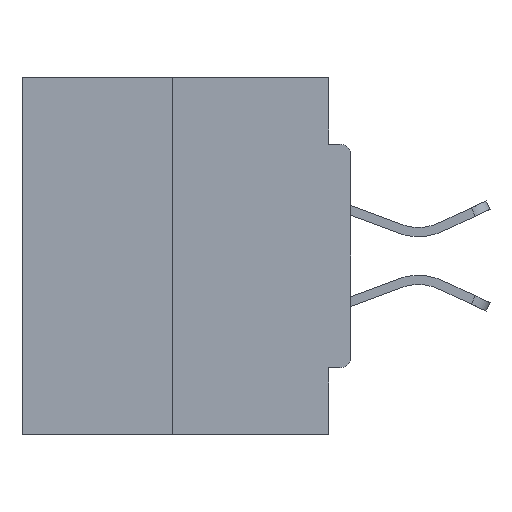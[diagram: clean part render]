
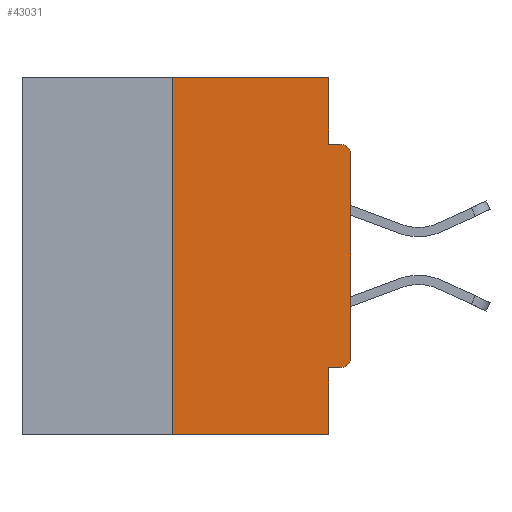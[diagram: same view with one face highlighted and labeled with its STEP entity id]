
A CAD part, left-side view. The second image highlights one B-rep face of the part: STEP entity #43031.
In plain terms, the highlighted planar face has unit normal (-1, 0, 0).
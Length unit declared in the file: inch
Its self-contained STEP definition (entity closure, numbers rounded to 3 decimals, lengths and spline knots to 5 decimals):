
#388 = EDGE_CURVE ( 'NONE', #30158, #618, #37627, .T. ) ;
#589 = EDGE_LOOP ( 'NONE', ( #16905, #14267, #35925, #22014, #29680, #1202, #29172, #22829, #21904, #15482 ) ) ;
#618 = VERTEX_POINT ( 'NONE', #36093 ) ;
#1078 = DIRECTION ( 'NONE',  ( 0., 0., -1. ) ) ;
#1202 = ORIENTED_EDGE ( 'NONE', *, *, #42570, .T. ) ;
#1735 = DIRECTION ( 'NONE',  ( 0., 1., 0. ) ) ;
#2717 = VERTEX_POINT ( 'NONE', #10126 ) ;
#3040 = VECTOR ( 'NONE', #42446, 39.37008 ) ;
#4078 = LINE ( 'NONE', #16279, #25141 ) ;
#4803 = DIRECTION ( 'NONE',  ( 0., 0., 1. ) ) ;
#5194 = CARTESIAN_POINT ( 'NONE',  ( 0., 0.031, -0.5 ) ) ;
#5253 = VERTEX_POINT ( 'NONE', #21710 ) ;
#5797 = VECTOR ( 'NONE', #20323, 39.37008 ) ;
#6685 = AXIS2_PLACEMENT_3D ( 'NONE', #8991, #26869, #28154 ) ;
#8008 = DIRECTION ( 'NONE',  ( -1., 0., 0. ) ) ;
#8043 = EDGE_CURVE ( 'NONE', #33575, #43270, #4078, .T. ) ;
#8541 = AXIS2_PLACEMENT_3D ( 'NONE', #38069, #44558, #27906 ) ;
#8991 = CARTESIAN_POINT ( 'NONE',  ( 0., 0.46, 0. ) ) ;
#9276 = CARTESIAN_POINT ( 'NONE',  ( 0., 0.031, 0. ) ) ;
#9399 = FACE_OUTER_BOUND ( 'NONE', #589, .T. ) ;
#9780 = DIRECTION ( 'NONE',  ( 0., -1., 0. ) ) ;
#10126 = CARTESIAN_POINT ( 'NONE',  ( 0., 0.031, 0. ) ) ;
#10431 = VECTOR ( 'NONE', #30221, 39.37008 ) ;
#10595 = VECTOR ( 'NONE', #38241, 39.37008 ) ;
#11610 = CARTESIAN_POINT ( 'NONE',  ( 0., 0., 0. ) ) ;
#12205 = CARTESIAN_POINT ( 'NONE',  ( 0., 0.25, -0.5 ) ) ;
#12233 = EDGE_CURVE ( 'NONE', #35413, #2717, #32429, .T. ) ;
#13070 = CARTESIAN_POINT ( 'NONE',  ( 0., 0.25, 0. ) ) ;
#14076 = CARTESIAN_POINT ( 'NONE',  ( 0., 0.031, -0.5 ) ) ;
#14267 = ORIENTED_EDGE ( 'NONE', *, *, #23577, .F. ) ;
#15436 = LINE ( 'NONE', #14076, #10595 ) ;
#15482 = ORIENTED_EDGE ( 'NONE', *, *, #19697, .F. ) ;
#15770 = CARTESIAN_POINT ( 'NONE',  ( 0., 0., -0.3915 ) ) ;
#16279 = CARTESIAN_POINT ( 'NONE',  ( 0., 0.46, -0.5 ) ) ;
#16905 = ORIENTED_EDGE ( 'NONE', *, *, #12233, .F. ) ;
#17288 = CIRCLE ( 'NONE', #37635, 0.015 ) ;
#17863 = VERTEX_POINT ( 'NONE', #33842 ) ;
#18727 = CARTESIAN_POINT ( 'NONE',  ( 0., 0.015, -0.3915 ) ) ;
#18904 = CARTESIAN_POINT ( 'NONE',  ( 0., 0.031, -0.0935 ) ) ;
#19132 = CARTESIAN_POINT ( 'NONE',  ( 0., 0.46, 0. ) ) ;
#19697 = EDGE_CURVE ( 'NONE', #2717, #30158, #44481, .T. ) ;
#20171 = CARTESIAN_POINT ( 'NONE',  ( 0., 0.015, -0.4065 ) ) ;
#20323 = DIRECTION ( 'NONE',  ( 0., 0., 1. ) ) ;
#21710 = CARTESIAN_POINT ( 'NONE',  ( 0., 0.031, -0.4065 ) ) ;
#21904 = ORIENTED_EDGE ( 'NONE', *, *, #388, .F. ) ;
#22014 = ORIENTED_EDGE ( 'NONE', *, *, #27966, .F. ) ;
#22829 = ORIENTED_EDGE ( 'NONE', *, *, #36757, .T. ) ;
#23577 = EDGE_CURVE ( 'NONE', #33575, #35413, #40900, .T. ) ;
#24592 = VERTEX_POINT ( 'NONE', #15770 ) ;
#25141 = VECTOR ( 'NONE', #9780, 39.37008 ) ;
#26398 = EDGE_CURVE ( 'NONE', #24592, #17863, #41490, .T. ) ;
#26869 = DIRECTION ( 'NONE',  ( 1., 0., 0. ) ) ;
#27906 = DIRECTION ( 'NONE',  ( 0., 0., -1. ) ) ;
#27966 = EDGE_CURVE ( 'NONE', #5253, #43270, #15436, .T. ) ;
#28154 = DIRECTION ( 'NONE',  ( 0., 0., -1. ) ) ;
#29172 = ORIENTED_EDGE ( 'NONE', *, *, #26398, .T. ) ;
#29680 = ORIENTED_EDGE ( 'NONE', *, *, #35485, .F. ) ;
#30158 = VERTEX_POINT ( 'NONE', #18904 ) ;
#30221 = DIRECTION ( 'NONE',  ( 0., 0., -1. ) ) ;
#31875 = CARTESIAN_POINT ( 'NONE',  ( 0., 0.25, 0. ) ) ;
#32097 = VECTOR ( 'NONE', #1735, 39.37008 ) ;
#32429 = LINE ( 'NONE', #19132, #40568 ) ;
#33575 = VERTEX_POINT ( 'NONE', #12205 ) ;
#33842 = CARTESIAN_POINT ( 'NONE',  ( 0., 0., -0.1085 ) ) ;
#35409 = LINE ( 'NONE', #39925, #32097 ) ;
#35413 = VERTEX_POINT ( 'NONE', #31875 ) ;
#35485 = EDGE_CURVE ( 'NONE', #40010, #5253, #35409, .T. ) ;
#35925 = ORIENTED_EDGE ( 'NONE', *, *, #8043, .T. ) ;
#36093 = CARTESIAN_POINT ( 'NONE',  ( 0., 0.015, -0.0935 ) ) ;
#36757 = EDGE_CURVE ( 'NONE', #17863, #618, #37456, .T. ) ;
#37456 = CIRCLE ( 'NONE', #8541, 0.015 ) ;
#37627 = LINE ( 'NONE', #42755, #3040 ) ;
#37635 = AXIS2_PLACEMENT_3D ( 'NONE', #18727, #8008, #1078 ) ;
#38069 = CARTESIAN_POINT ( 'NONE',  ( 0., 0.015, -0.1085 ) ) ;
#38241 = DIRECTION ( 'NONE',  ( 0., 0., -1. ) ) ;
#39925 = CARTESIAN_POINT ( 'NONE',  ( 0., 0., -0.4065 ) ) ;
#40010 = VERTEX_POINT ( 'NONE', #20171 ) ;
#40413 = VECTOR ( 'NONE', #4803, 39.37008 ) ;
#40568 = VECTOR ( 'NONE', #43400, 39.37008 ) ;
#40900 = LINE ( 'NONE', #13070, #5797 ) ;
#41490 = LINE ( 'NONE', #11610, #40413 ) ;
#42434 = PLANE ( 'NONE',  #6685 ) ;
#42446 = DIRECTION ( 'NONE',  ( 0., -1., 0. ) ) ;
#42570 = EDGE_CURVE ( 'NONE', #40010, #24592, #17288, .T. ) ;
#42755 = CARTESIAN_POINT ( 'NONE',  ( 0., 0., -0.0935 ) ) ;
#43031 = ADVANCED_FACE ( 'NONE', ( #9399 ), #42434, .F. ) ;
#43270 = VERTEX_POINT ( 'NONE', #5194 ) ;
#43400 = DIRECTION ( 'NONE',  ( 0., -1., 0. ) ) ;
#44481 = LINE ( 'NONE', #9276, #10431 ) ;
#44558 = DIRECTION ( 'NONE',  ( -1., 0., 0. ) ) ;
